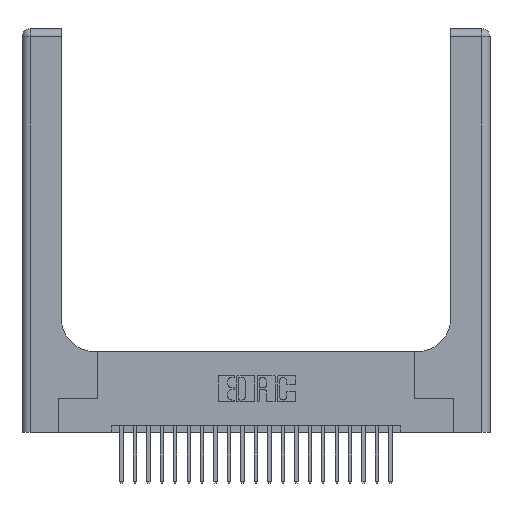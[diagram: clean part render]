
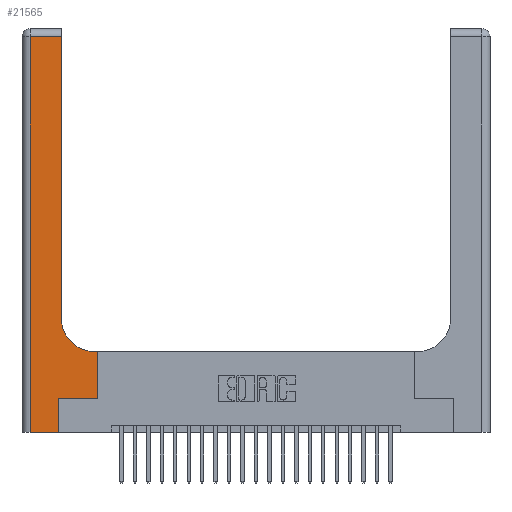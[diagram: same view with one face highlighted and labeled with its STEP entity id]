
A CAD part, top view. The second image highlights one B-rep face of the part: STEP entity #21565.
In plain terms, the highlighted planar face has unit normal (0, 0, 1).
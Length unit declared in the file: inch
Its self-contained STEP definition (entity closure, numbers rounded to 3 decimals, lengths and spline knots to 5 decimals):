
#83 = EDGE_CURVE ( 'NONE', #23940, #17486, #3378, .T. ) ;
#568 = VERTEX_POINT ( 'NONE', #12653 ) ;
#609 = VECTOR ( 'NONE', #20402, 39.37008 ) ;
#970 = LINE ( 'NONE', #13291, #21160 ) ;
#1029 = EDGE_CURVE ( 'NONE', #15137, #16924, #19336, .T. ) ;
#1048 = AXIS2_PLACEMENT_3D ( 'NONE', #22023, #10821, #23885 ) ;
#1381 = CARTESIAN_POINT ( 'NONE',  ( 0.2915, 0.85, 0.37 ) ) ;
#1935 = DIRECTION ( 'NONE',  ( -1., 0., 0. ) ) ;
#2422 = CARTESIAN_POINT ( 'NONE',  ( 0.5415, 0.6, 0.37 ) ) ;
#3239 = CARTESIAN_POINT ( 'NONE',  ( 0.5585, 0.6, 0.37 ) ) ;
#3378 = LINE ( 'NONE', #7610, #16773 ) ;
#4026 = DIRECTION ( 'NONE',  ( 0., 0., -1. ) ) ;
#4352 = EDGE_CURVE ( 'NONE', #12284, #568, #18969, .T. ) ;
#4897 = CARTESIAN_POINT ( 'NONE',  ( 0.269, 0., 0.37 ) ) ;
#5119 = VERTEX_POINT ( 'NONE', #11747 ) ;
#5252 = CARTESIAN_POINT ( 'NONE',  ( 0.06, 3., 0.37 ) ) ;
#5476 = LINE ( 'NONE', #6840, #19403 ) ;
#6101 = DIRECTION ( 'NONE',  ( 1., 0., 0. ) ) ;
#6140 = VECTOR ( 'NONE', #14435, 39.37008 ) ;
#6350 = LINE ( 'NONE', #5252, #609 ) ;
#6442 = EDGE_LOOP ( 'NONE', ( #17080, #19407, #11810, #23467, #10311, #17669, #11231, #10023, #20336 ) ) ;
#6753 = LINE ( 'NONE', #4897, #6140 ) ;
#6840 = CARTESIAN_POINT ( 'NONE',  ( 0.2915, 3., 0.37 ) ) ;
#7537 = VECTOR ( 'NONE', #6101, 39.37008 ) ;
#7610 = CARTESIAN_POINT ( 'NONE',  ( 0.2915, 0.6, 0.37 ) ) ;
#7749 = DIRECTION ( 'NONE',  ( -1., 0., 0. ) ) ;
#7751 = EDGE_CURVE ( 'NONE', #16924, #23940, #970, .T. ) ;
#8426 = EDGE_CURVE ( 'NONE', #5119, #13363, #12684, .T. ) ;
#8489 = CARTESIAN_POINT ( 'NONE',  ( 0.269, 0., 0.37 ) ) ;
#10023 = ORIENTED_EDGE ( 'NONE', *, *, #83, .T. ) ;
#10261 = CARTESIAN_POINT ( 'NONE',  ( 0.269, 0.25, 0.37 ) ) ;
#10311 = ORIENTED_EDGE ( 'NONE', *, *, #24453, .T. ) ;
#10351 = DIRECTION ( 'NONE',  ( 1., 0., 0. ) ) ;
#10821 = DIRECTION ( 'NONE',  ( 0., 0., -1. ) ) ;
#11231 = ORIENTED_EDGE ( 'NONE', *, *, #7751, .T. ) ;
#11747 = CARTESIAN_POINT ( 'NONE',  ( 0.06, 0., 0.37 ) ) ;
#11797 = EDGE_CURVE ( 'NONE', #21648, #12284, #5476, .T. ) ;
#11810 = ORIENTED_EDGE ( 'NONE', *, *, #18824, .T. ) ;
#12284 = VERTEX_POINT ( 'NONE', #14171 ) ;
#12653 = CARTESIAN_POINT ( 'NONE',  ( 0.06, 2.94, 0.37 ) ) ;
#12684 = LINE ( 'NONE', #15605, #7537 ) ;
#13291 = CARTESIAN_POINT ( 'NONE',  ( 0.5585, 0.25, 0.37 ) ) ;
#13363 = VERTEX_POINT ( 'NONE', #8489 ) ;
#13814 = EDGE_CURVE ( 'NONE', #17486, #21648, #15227, .T. ) ;
#14171 = CARTESIAN_POINT ( 'NONE',  ( 0.2915, 2.94, 0.37 ) ) ;
#14401 = VECTOR ( 'NONE', #10351, 39.37008 ) ;
#14435 = DIRECTION ( 'NONE',  ( 0., 1., 0. ) ) ;
#15137 = VERTEX_POINT ( 'NONE', #17593 ) ;
#15176 = DIRECTION ( 'NONE',  ( 0., 1., 0. ) ) ;
#15227 = CIRCLE ( 'NONE', #18804, 0.25 ) ;
#15445 = CARTESIAN_POINT ( 'NONE',  ( 0.5415, 0.85, 0.37 ) ) ;
#15605 = CARTESIAN_POINT ( 'NONE',  ( 0., 0., 0.37 ) ) ;
#15721 = CARTESIAN_POINT ( 'NONE',  ( 0., 2.94, 0.37 ) ) ;
#16773 = VECTOR ( 'NONE', #7749, 39.37008 ) ;
#16924 = VERTEX_POINT ( 'NONE', #17914 ) ;
#17080 = ORIENTED_EDGE ( 'NONE', *, *, #11797, .T. ) ;
#17332 = DIRECTION ( 'NONE',  ( 1., 0., 0. ) ) ;
#17486 = VERTEX_POINT ( 'NONE', #2422 ) ;
#17593 = CARTESIAN_POINT ( 'NONE',  ( 0.269, 0.25, 0.37 ) ) ;
#17669 = ORIENTED_EDGE ( 'NONE', *, *, #1029, .T. ) ;
#17914 = CARTESIAN_POINT ( 'NONE',  ( 0.5585, 0.25, 0.37 ) ) ;
#18385 = VECTOR ( 'NONE', #1935, 39.37008 ) ;
#18804 = AXIS2_PLACEMENT_3D ( 'NONE', #15445, #4026, #17332 ) ;
#18824 = EDGE_CURVE ( 'NONE', #568, #5119, #6350, .T. ) ;
#18969 = LINE ( 'NONE', #15721, #18385 ) ;
#19336 = LINE ( 'NONE', #10261, #14401 ) ;
#19403 = VECTOR ( 'NONE', #23699, 39.37008 ) ;
#19407 = ORIENTED_EDGE ( 'NONE', *, *, #4352, .T. ) ;
#20156 = PLANE ( 'NONE',  #1048 ) ;
#20336 = ORIENTED_EDGE ( 'NONE', *, *, #13814, .T. ) ;
#20402 = DIRECTION ( 'NONE',  ( 0., -1., 0. ) ) ;
#21160 = VECTOR ( 'NONE', #15176, 39.37008 ) ;
#21565 = ADVANCED_FACE ( 'NONE', ( #22449 ), #20156, .F. ) ;
#21648 = VERTEX_POINT ( 'NONE', #1381 ) ;
#22023 = CARTESIAN_POINT ( 'NONE',  ( 0., 3., 0.37 ) ) ;
#22449 = FACE_OUTER_BOUND ( 'NONE', #6442, .T. ) ;
#23467 = ORIENTED_EDGE ( 'NONE', *, *, #8426, .T. ) ;
#23699 = DIRECTION ( 'NONE',  ( 0., 1., 0. ) ) ;
#23885 = DIRECTION ( 'NONE',  ( -1., 0., 0. ) ) ;
#23940 = VERTEX_POINT ( 'NONE', #3239 ) ;
#24453 = EDGE_CURVE ( 'NONE', #13363, #15137, #6753, .T. ) ;
